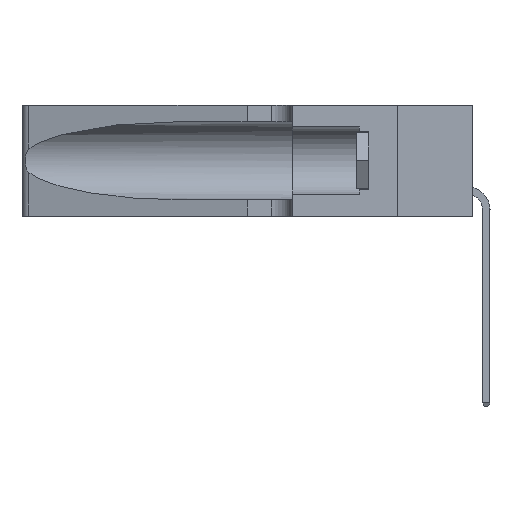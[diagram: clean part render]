
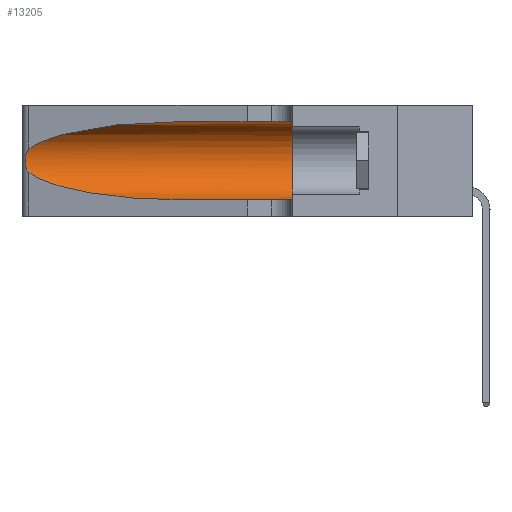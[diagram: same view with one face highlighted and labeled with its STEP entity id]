
A CAD part, left-side view. The second image highlights one B-rep face of the part: STEP entity #13205.
In plain terms, the highlighted cylindrical face has radius 3.308 mm (diameter 6.617 mm), a partial arc.
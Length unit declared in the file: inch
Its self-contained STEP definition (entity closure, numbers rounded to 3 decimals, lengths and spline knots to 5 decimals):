
#224 = VERTEX_POINT ( 'NONE', #10354 ) ;
#569 = CARTESIAN_POINT ( 'NONE',  ( 0.2373, 1.15595, 0.08982 ) ) ;
#1792 = B_SPLINE_CURVE_WITH_KNOTS ( 'NONE', 3,
 ( #30943, #34486, #20487, #12460, #16467, #38171, #16630, #16144, #23573, #38649, #38326, #20158, #45776, #23896 ),
 .UNSPECIFIED., .F., .F.,
 ( 4, 2, 2, 2, 2, 2, 4 ),
 ( 0., 0.00027, 0.00053, 0.00107, 0.0016, 0.00187, 0.00214 ),
 .UNSPECIFIED. ) ;
#2848 = VERTEX_POINT ( 'NONE', #42549 ) ;
#4531 = ORIENTED_EDGE ( 'NONE', *, *, #42004, .T. ) ;
#4907 = CARTESIAN_POINT ( 'NONE',  ( 0.1305, 1.61858, 0.185 ) ) ;
#5052 = CIRCLE ( 'NONE', #7498, 0.13025 ) ;
#6661 = CARTESIAN_POINT ( 'NONE',  ( 0.2373, 1.15595, 0.28018 ) ) ;
#6935 = EDGE_CURVE ( 'NONE', #29165, #13372, #1792, .T. ) ;
#7498 = AXIS2_PLACEMENT_3D ( 'NONE', #36919, #18942, #44536 ) ;
#10354 = CARTESIAN_POINT ( 'NONE',  ( 0.1305, 0.35, 0.05475 ) ) ;
#10363 = DIRECTION ( 'NONE',  ( 0., -1., 0. ) ) ;
#10863 =( BOUNDED_CURVE ( )  B_SPLINE_CURVE ( 3, ( #42707, #36032, #6661, #46390 ),
 .UNSPECIFIED., .F., .F. ) 
 B_SPLINE_CURVE_WITH_KNOTS ( ( 4, 4 ),
 ( 1.5708, 2.84003 ),
 .UNSPECIFIED. ) 
 CURVE ( )  GEOMETRIC_REPRESENTATION_ITEM ( )  RATIONAL_B_SPLINE_CURVE ( ( 1., 0.87, 0.87, 1. ) ) 
 REPRESENTATION_ITEM ( '' )  );
#12236 = DIRECTION ( 'NONE',  ( 0., -1., 0. ) ) ;
#12382 = AXIS2_PLACEMENT_3D ( 'NONE', #4907, #12236, #34413 ) ;
#12460 = CARTESIAN_POINT ( 'NONE',  ( 0.25787, 1.23484, 0.2124 ) ) ;
#13205 = ADVANCED_FACE ( 'NONE', ( #23460 ), #18825, .F. ) ;
#13372 = VERTEX_POINT ( 'NONE', #24465 ) ;
#13637 = EDGE_CURVE ( 'NONE', #2848, #224, #5052, .T. ) ;
#16144 = CARTESIAN_POINT ( 'NONE',  ( 0.26075, 1.23896, 0.178 ) ) ;
#16467 = CARTESIAN_POINT ( 'NONE',  ( 0.25854, 1.2359, 0.20912 ) ) ;
#16630 = CARTESIAN_POINT ( 'NONE',  ( 0.26075, 1.23896, 0.19203 ) ) ;
#18825 = CYLINDRICAL_SURFACE ( 'NONE', #12382, 0.13025 ) ;
#18942 = DIRECTION ( 'NONE',  ( 0., 1., 0. ) ) ;
#20158 = CARTESIAN_POINT ( 'NONE',  ( 0.25639, 1.23186, 0.15144 ) ) ;
#20459 = ORIENTED_EDGE ( 'NONE', *, *, #37686, .T. ) ;
#20487 = CARTESIAN_POINT ( 'NONE',  ( 0.25639, 1.23184, 0.21858 ) ) ;
#21914 = CARTESIAN_POINT ( 'NONE',  ( 0.1305, 0.72297, 0.31525 ) ) ;
#22371 = CARTESIAN_POINT ( 'NONE',  ( 0.18966, 0.96281, 0.05475 ) ) ;
#23460 = FACE_OUTER_BOUND ( 'NONE', #27889, .T. ) ;
#23573 = CARTESIAN_POINT ( 'NONE',  ( 0.26017, 1.23833, 0.17102 ) ) ;
#23896 = CARTESIAN_POINT ( 'NONE',  ( 0.25487, 1.22718, 0.14631 ) ) ;
#24465 = CARTESIAN_POINT ( 'NONE',  ( 0.25487, 1.22718, 0.14631 ) ) ;
#24602 = VERTEX_POINT ( 'NONE', #45015 ) ;
#26809 = CARTESIAN_POINT ( 'NONE',  ( 0.25487, 1.22718, 0.22369 ) ) ;
#26953 = ORIENTED_EDGE ( 'NONE', *, *, #6935, .T. ) ;
#27181 = DIRECTION ( 'NONE',  ( 0., -1., 0. ) ) ;
#27889 = EDGE_LOOP ( 'NONE', ( #4531, #26953, #34303, #20459, #41710, #38614 ) ) ;
#28363 = EDGE_CURVE ( 'NONE', #13372, #24602, #35913, .T. ) ;
#29165 = VERTEX_POINT ( 'NONE', #26809 ) ;
#30943 = CARTESIAN_POINT ( 'NONE',  ( 0.25487, 1.22718, 0.22369 ) ) ;
#31231 = VERTEX_POINT ( 'NONE', #21914 ) ;
#33447 = EDGE_CURVE ( 'NONE', #31231, #2848, #46373, .T. ) ;
#34303 = ORIENTED_EDGE ( 'NONE', *, *, #28363, .T. ) ;
#34413 = DIRECTION ( 'NONE',  ( 0., 0., -1. ) ) ;
#34486 = CARTESIAN_POINT ( 'NONE',  ( 0.25555, 1.22994, 0.2215 ) ) ;
#34842 = LINE ( 'NONE', #47050, #44491 ) ;
#35913 =( BOUNDED_CURVE ( )  B_SPLINE_CURVE ( 3, ( #37438, #569, #22371, #40465 ),
 .UNSPECIFIED., .F., .F. ) 
 B_SPLINE_CURVE_WITH_KNOTS ( ( 4, 4 ),
 ( 3.44316, 4.71239 ),
 .UNSPECIFIED. ) 
 CURVE ( )  GEOMETRIC_REPRESENTATION_ITEM ( )  RATIONAL_B_SPLINE_CURVE ( ( 1., 0.87, 0.87, 1. ) ) 
 REPRESENTATION_ITEM ( '' )  );
#36032 = CARTESIAN_POINT ( 'NONE',  ( 0.18966, 0.96281, 0.31525 ) ) ;
#36919 = CARTESIAN_POINT ( 'NONE',  ( 0.1305, 0.35, 0.185 ) ) ;
#37438 = CARTESIAN_POINT ( 'NONE',  ( 0.25487, 1.22718, 0.14631 ) ) ;
#37686 = EDGE_CURVE ( 'NONE', #24602, #224, #34842, .T. ) ;
#37748 = CARTESIAN_POINT ( 'NONE',  ( 0.1305, 1.61858, 0.31525 ) ) ;
#38171 = CARTESIAN_POINT ( 'NONE',  ( 0.26018, 1.23835, 0.19895 ) ) ;
#38326 = CARTESIAN_POINT ( 'NONE',  ( 0.25789, 1.23486, 0.15765 ) ) ;
#38614 = ORIENTED_EDGE ( 'NONE', *, *, #33447, .F. ) ;
#38649 = CARTESIAN_POINT ( 'NONE',  ( 0.25856, 1.23593, 0.16098 ) ) ;
#40465 = CARTESIAN_POINT ( 'NONE',  ( 0.1305, 0.72297, 0.05475 ) ) ;
#41710 = ORIENTED_EDGE ( 'NONE', *, *, #13637, .F. ) ;
#41779 = VECTOR ( 'NONE', #27181, 39.37008 ) ;
#42004 = EDGE_CURVE ( 'NONE', #31231, #29165, #10863, .T. ) ;
#42549 = CARTESIAN_POINT ( 'NONE',  ( 0.1305, 0.35, 0.31525 ) ) ;
#42707 = CARTESIAN_POINT ( 'NONE',  ( 0.1305, 0.72297, 0.31525 ) ) ;
#44491 = VECTOR ( 'NONE', #10363, 39.37008 ) ;
#44536 = DIRECTION ( 'NONE',  ( 0., 0., 1. ) ) ;
#45015 = CARTESIAN_POINT ( 'NONE',  ( 0.1305, 0.72297, 0.05475 ) ) ;
#45776 = CARTESIAN_POINT ( 'NONE',  ( 0.25555, 1.22993, 0.14849 ) ) ;
#46373 = LINE ( 'NONE', #37748, #41779 ) ;
#46390 = CARTESIAN_POINT ( 'NONE',  ( 0.25487, 1.22718, 0.22369 ) ) ;
#47050 = CARTESIAN_POINT ( 'NONE',  ( 0.1305, 1.61858, 0.05475 ) ) ;
